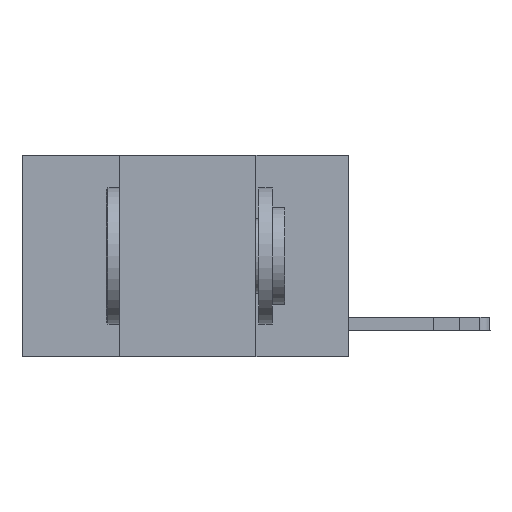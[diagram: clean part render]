
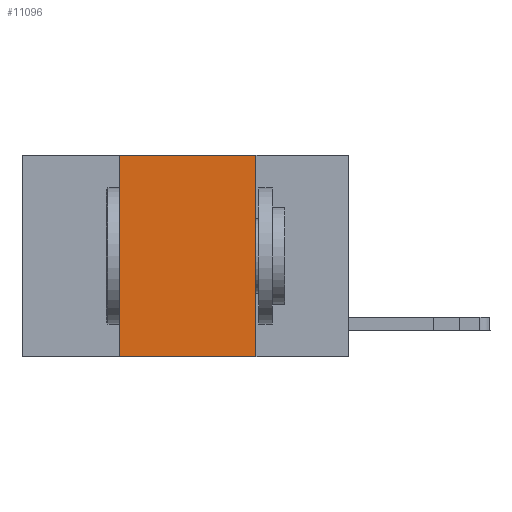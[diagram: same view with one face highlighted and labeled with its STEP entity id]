
A CAD part, left-side view. The second image highlights one B-rep face of the part: STEP entity #11096.
In plain terms, the highlighted planar face has unit normal (-1, 0, 0).
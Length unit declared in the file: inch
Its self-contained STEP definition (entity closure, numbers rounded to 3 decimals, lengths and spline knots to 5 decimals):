
#580 = VERTEX_POINT ( 'NONE', #642 ) ;
#642 = CARTESIAN_POINT ( 'NONE',  ( 0., 0.17, 0. ) ) ;
#951 = DIRECTION ( 'NONE',  ( 0., 0., 1. ) ) ;
#992 = ORIENTED_EDGE ( 'NONE', *, *, #14406, .F. ) ;
#1013 = DIRECTION ( 'NONE',  ( 1., 0., 0. ) ) ;
#1399 = ORIENTED_EDGE ( 'NONE', *, *, #13622, .T. ) ;
#3701 = DIRECTION ( 'NONE',  ( 0., 0., -1. ) ) ;
#3769 = LINE ( 'NONE', #14747, #10956 ) ;
#4411 = DIRECTION ( 'NONE',  ( 0., -1., 0. ) ) ;
#4496 = LINE ( 'NONE', #15344, #13623 ) ;
#4530 = LINE ( 'NONE', #13930, #10181 ) ;
#4840 = AXIS2_PLACEMENT_3D ( 'NONE', #8411, #1013, #9603 ) ;
#5279 = CARTESIAN_POINT ( 'NONE',  ( 0., 0.42, 0. ) ) ;
#6021 = VECTOR ( 'NONE', #3701, 39.37008 ) ;
#6154 = CARTESIAN_POINT ( 'NONE',  ( 0., 0.17, 0. ) ) ;
#6384 = VERTEX_POINT ( 'NONE', #5279 ) ;
#6402 = EDGE_CURVE ( 'NONE', #6384, #580, #3769, .T. ) ;
#6493 = DIRECTION ( 'NONE',  ( 0., -1., 0. ) ) ;
#6889 = FACE_OUTER_BOUND ( 'NONE', #7578, .T. ) ;
#7578 = EDGE_LOOP ( 'NONE', ( #13098, #10350, #992, #1399 ) ) ;
#8411 = CARTESIAN_POINT ( 'NONE',  ( 0., 0.6, 0. ) ) ;
#9603 = DIRECTION ( 'NONE',  ( 0., 0., -1. ) ) ;
#9953 = LINE ( 'NONE', #6154, #6021 ) ;
#10181 = VECTOR ( 'NONE', #4411, 39.37008 ) ;
#10350 = ORIENTED_EDGE ( 'NONE', *, *, #6402, .F. ) ;
#10749 = CARTESIAN_POINT ( 'NONE',  ( 0., 0.42, -0.37 ) ) ;
#10956 = VECTOR ( 'NONE', #6493, 39.37008 ) ;
#11096 = ADVANCED_FACE ( 'NONE', ( #6889 ), #14225, .F. ) ;
#12724 = CARTESIAN_POINT ( 'NONE',  ( 0., 0.17, -0.37 ) ) ;
#13024 = VERTEX_POINT ( 'NONE', #12724 ) ;
#13098 = ORIENTED_EDGE ( 'NONE', *, *, #15183, .F. ) ;
#13110 = VERTEX_POINT ( 'NONE', #10749 ) ;
#13622 = EDGE_CURVE ( 'NONE', #13110, #13024, #4530, .T. ) ;
#13623 = VECTOR ( 'NONE', #951, 39.37008 ) ;
#13930 = CARTESIAN_POINT ( 'NONE',  ( 0., 0.6, -0.37 ) ) ;
#14225 = PLANE ( 'NONE',  #4840 ) ;
#14406 = EDGE_CURVE ( 'NONE', #13110, #6384, #4496, .T. ) ;
#14747 = CARTESIAN_POINT ( 'NONE',  ( 0., 0.6, 0. ) ) ;
#15183 = EDGE_CURVE ( 'NONE', #580, #13024, #9953, .T. ) ;
#15344 = CARTESIAN_POINT ( 'NONE',  ( 0., 0.42, 0. ) ) ;
